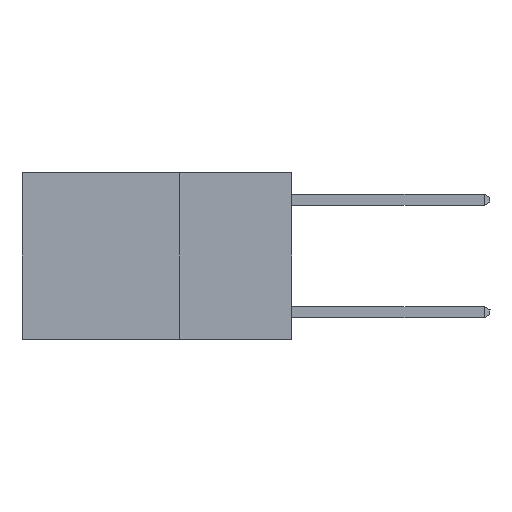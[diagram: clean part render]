
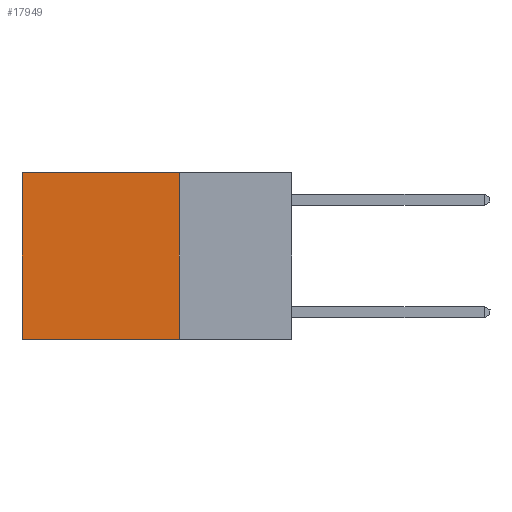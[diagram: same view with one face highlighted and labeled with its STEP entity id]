
A CAD part, left-side view. The second image highlights one B-rep face of the part: STEP entity #17949.
In plain terms, the highlighted planar face has unit normal (-1, 0, 0).
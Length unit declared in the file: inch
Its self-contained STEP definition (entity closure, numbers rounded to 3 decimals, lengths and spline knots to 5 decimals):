
#823 = CARTESIAN_POINT ( 'NONE',  ( 0.2625, 0.6, -0.37 ) ) ;
#1430 = ORIENTED_EDGE ( 'NONE', *, *, #5832, .F. ) ;
#1543 = CARTESIAN_POINT ( 'NONE',  ( 0.2625, 0.25, -0.37 ) ) ;
#1734 = VECTOR ( 'NONE', #25897, 39.37008 ) ;
#2641 = EDGE_CURVE ( 'NONE', #18134, #25187, #28193, .T. ) ;
#4851 = AXIS2_PLACEMENT_3D ( 'NONE', #9990, #19354, #5409 ) ;
#5179 = CARTESIAN_POINT ( 'NONE',  ( 0.2625, 0.25, -0.37 ) ) ;
#5409 = DIRECTION ( 'NONE',  ( 0., 0., -1. ) ) ;
#5540 = CARTESIAN_POINT ( 'NONE',  ( 0.2625, 0.25, 0. ) ) ;
#5832 = EDGE_CURVE ( 'NONE', #21987, #20772, #29418, .T. ) ;
#7326 = CARTESIAN_POINT ( 'NONE',  ( 0.2625, 0.25, 0. ) ) ;
#7527 = DIRECTION ( 'NONE',  ( 0., 1., 0. ) ) ;
#8346 = DIRECTION ( 'NONE',  ( 0., 0., -1. ) ) ;
#8464 = CARTESIAN_POINT ( 'NONE',  ( 0.2625, 0.6, 0. ) ) ;
#8719 = LINE ( 'NONE', #7326, #1734 ) ;
#9253 = CARTESIAN_POINT ( 'NONE',  ( 0.2625, 0.25, 0. ) ) ;
#9990 = CARTESIAN_POINT ( 'NONE',  ( 0.2625, 0.25, 0. ) ) ;
#10325 = DIRECTION ( 'NONE',  ( 0., 0., -1. ) ) ;
#12671 = ORIENTED_EDGE ( 'NONE', *, *, #29679, .T. ) ;
#13185 = EDGE_LOOP ( 'NONE', ( #13490, #22548, #1430, #12671 ) ) ;
#13490 = ORIENTED_EDGE ( 'NONE', *, *, #2641, .T. ) ;
#15125 = FACE_OUTER_BOUND ( 'NONE', #13185, .T. ) ;
#17016 = PLANE ( 'NONE',  #4851 ) ;
#17705 = CARTESIAN_POINT ( 'NONE',  ( 0.2625, 0.6, 0. ) ) ;
#17949 = ADVANCED_FACE ( 'NONE', ( #15125 ), #17016, .F. ) ;
#18134 = VERTEX_POINT ( 'NONE', #8464 ) ;
#19354 = DIRECTION ( 'NONE',  ( 1., 0., 0. ) ) ;
#20772 = VERTEX_POINT ( 'NONE', #1543 ) ;
#21632 = EDGE_CURVE ( 'NONE', #20772, #25187, #25683, .T. ) ;
#21987 = VERTEX_POINT ( 'NONE', #9253 ) ;
#22134 = VECTOR ( 'NONE', #7527, 39.37008 ) ;
#22548 = ORIENTED_EDGE ( 'NONE', *, *, #21632, .F. ) ;
#25187 = VERTEX_POINT ( 'NONE', #823 ) ;
#25683 = LINE ( 'NONE', #5179, #22134 ) ;
#25897 = DIRECTION ( 'NONE',  ( 0., 1., 0. ) ) ;
#26797 = VECTOR ( 'NONE', #8346, 39.37008 ) ;
#28010 = VECTOR ( 'NONE', #10325, 39.37008 ) ;
#28193 = LINE ( 'NONE', #17705, #26797 ) ;
#29418 = LINE ( 'NONE', #5540, #28010 ) ;
#29679 = EDGE_CURVE ( 'NONE', #21987, #18134, #8719, .T. ) ;
